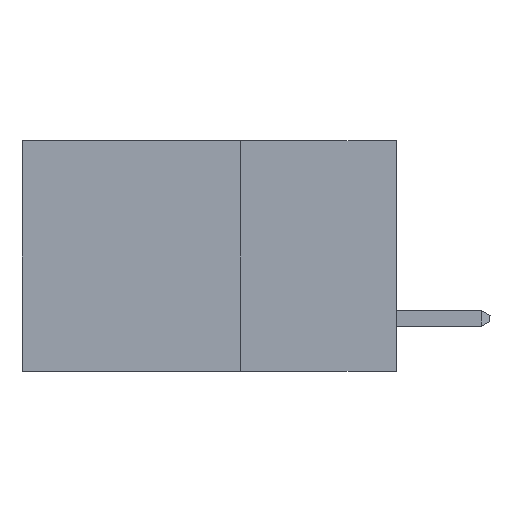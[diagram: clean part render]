
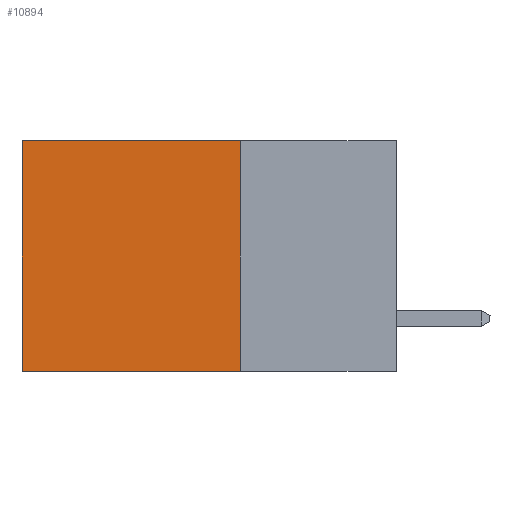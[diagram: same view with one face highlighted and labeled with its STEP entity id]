
A CAD part, left-side view. The second image highlights one B-rep face of the part: STEP entity #10894.
In plain terms, the highlighted planar face has unit normal (-1, 0, 0).
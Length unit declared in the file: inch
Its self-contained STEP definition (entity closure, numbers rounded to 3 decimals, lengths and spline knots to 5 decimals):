
#220 = CARTESIAN_POINT ( 'NONE',  ( 0.2615, 0.6, -0.37 ) ) ;
#1712 = VECTOR ( 'NONE', #15912, 39.37008 ) ;
#1736 = AXIS2_PLACEMENT_3D ( 'NONE', #10442, #13310, #11870 ) ;
#1778 = CARTESIAN_POINT ( 'NONE',  ( 0.2615, 0.6, -0.37 ) ) ;
#2294 = CARTESIAN_POINT ( 'NONE',  ( 0.2615, 0.25, -0.37 ) ) ;
#2840 = EDGE_CURVE ( 'NONE', #4618, #3471, #5959, .T. ) ;
#3471 = VERTEX_POINT ( 'NONE', #1778 ) ;
#3728 = VERTEX_POINT ( 'NONE', #8295 ) ;
#3866 = EDGE_CURVE ( 'NONE', #3728, #3471, #13395, .T. ) ;
#4618 = VERTEX_POINT ( 'NONE', #2294 ) ;
#4826 = LINE ( 'NONE', #10698, #14656 ) ;
#5556 = ORIENTED_EDGE ( 'NONE', *, *, #11681, .T. ) ;
#5781 = CARTESIAN_POINT ( 'NONE',  ( 0.2615, 0.25, -0.37 ) ) ;
#5959 = LINE ( 'NONE', #14937, #11166 ) ;
#6942 = LINE ( 'NONE', #5781, #1712 ) ;
#8295 = CARTESIAN_POINT ( 'NONE',  ( 0.2615, 0.6, 0. ) ) ;
#9819 = ORIENTED_EDGE ( 'NONE', *, *, #3866, .T. ) ;
#10062 = EDGE_CURVE ( 'NONE', #15432, #4618, #6942, .T. ) ;
#10163 = PLANE ( 'NONE',  #1736 ) ;
#10442 = CARTESIAN_POINT ( 'NONE',  ( 0.2615, 0.25, -0.37 ) ) ;
#10532 = CARTESIAN_POINT ( 'NONE',  ( 0.2615, 0.25, 0. ) ) ;
#10698 = CARTESIAN_POINT ( 'NONE',  ( 0.2615, 0.25, 0. ) ) ;
#10878 = DIRECTION ( 'NONE',  ( 0., 1., 0. ) ) ;
#10894 = ADVANCED_FACE ( 'NONE', ( #11763 ), #10163, .F. ) ;
#11166 = VECTOR ( 'NONE', #17707, 39.37008 ) ;
#11681 = EDGE_CURVE ( 'NONE', #15432, #3728, #4826, .T. ) ;
#11763 = FACE_OUTER_BOUND ( 'NONE', #14120, .T. ) ;
#11870 = DIRECTION ( 'NONE',  ( 0., 0., -1. ) ) ;
#12949 = ORIENTED_EDGE ( 'NONE', *, *, #10062, .F. ) ;
#13310 = DIRECTION ( 'NONE',  ( 1., 0., 0. ) ) ;
#13395 = LINE ( 'NONE', #220, #16728 ) ;
#13489 = DIRECTION ( 'NONE',  ( 0., 0., -1. ) ) ;
#14120 = EDGE_LOOP ( 'NONE', ( #9819, #16030, #12949, #5556 ) ) ;
#14656 = VECTOR ( 'NONE', #10878, 39.37008 ) ;
#14937 = CARTESIAN_POINT ( 'NONE',  ( 0.2615, 0.25, -0.37 ) ) ;
#15432 = VERTEX_POINT ( 'NONE', #10532 ) ;
#15912 = DIRECTION ( 'NONE',  ( 0., 0., -1. ) ) ;
#16030 = ORIENTED_EDGE ( 'NONE', *, *, #2840, .F. ) ;
#16728 = VECTOR ( 'NONE', #13489, 39.37008 ) ;
#17707 = DIRECTION ( 'NONE',  ( 0., 1., 0. ) ) ;
